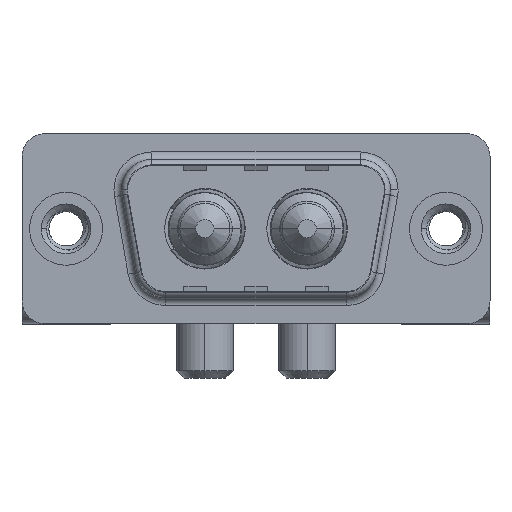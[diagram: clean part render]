
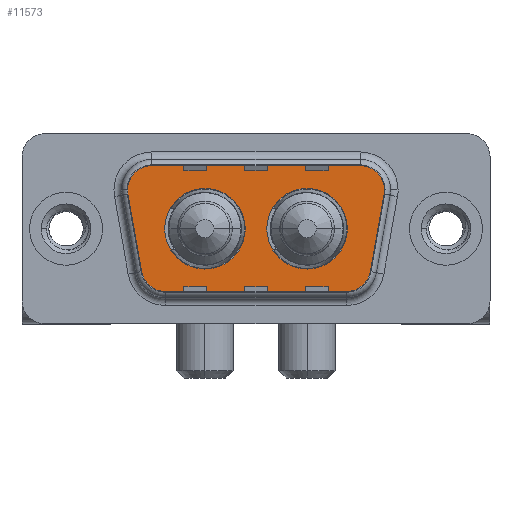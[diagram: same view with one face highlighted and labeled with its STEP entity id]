
A CAD part, top view. The second image highlights one B-rep face of the part: STEP entity #11573.
In plain terms, the highlighted planar face has unit normal (0, 0, 1).
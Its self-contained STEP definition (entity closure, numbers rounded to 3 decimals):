
#195 = EDGE_CURVE ( 'NONE', #11482, #9476, #1524, .T. ) ;
#205 = EDGE_CURVE ( 'NONE', #4298, #3397, #11336, .T. ) ;
#238 = VERTEX_POINT ( 'NONE', #2735 ) ;
#499 = LINE ( 'NONE', #4346, #11280 ) ;
#601 = LINE ( 'NONE', #11205, #11908 ) ;
#615 = LINE ( 'NONE', #6874, #2992 ) ;
#652 = DIRECTION ( 'NONE',  ( 1., 0., 0. ) ) ;
#733 = ORIENTED_EDGE ( 'NONE', *, *, #5882, .T. ) ;
#870 = EDGE_CURVE ( 'NONE', #4586, #8740, #4844, .T. ) ;
#877 = EDGE_LOOP ( 'NONE', ( #5387, #3769 ) ) ;
#968 = EDGE_CURVE ( 'NONE', #10297, #6879, #2413, .T. ) ;
#1195 = ORIENTED_EDGE ( 'NONE', *, *, #8867, .T. ) ;
#1219 = CARTESIAN_POINT ( 'NONE',  ( 5.436, 4.9, 0. ) ) ;
#1524 = LINE ( 'NONE', #3479, #8083 ) ;
#1989 = AXIS2_PLACEMENT_3D ( 'NONE', #2978, #10566, #10689 ) ;
#2013 = CARTESIAN_POINT ( 'NONE',  ( 21.534, 2.553, 0. ) ) ;
#2073 = DIRECTION ( 'NONE',  ( 0., 0., 1. ) ) ;
#2329 = ORIENTED_EDGE ( 'NONE', *, *, #8254, .T. ) ;
#2391 = DIRECTION ( 'NONE',  ( 1., 0., 0. ) ) ;
#2413 = CIRCLE ( 'NONE', #5630, 2.65 ) ;
#2735 = CARTESIAN_POINT ( 'NONE',  ( 6.459, -4.9, 0. ) ) ;
#2789 = ORIENTED_EDGE ( 'NONE', *, *, #870, .F. ) ;
#2978 = CARTESIAN_POINT ( 'NONE',  ( 18.541, -2.9, 0. ) ) ;
#2992 = VECTOR ( 'NONE', #12122, 1000. ) ;
#3397 = VERTEX_POINT ( 'NONE', #11050 ) ;
#3421 = DIRECTION ( 'NONE',  ( 0., 0., 1. ) ) ;
#3461 = DIRECTION ( 'NONE',  ( 0., 0., 1. ) ) ;
#3479 = CARTESIAN_POINT ( 'NONE',  ( 3.466, 2.553, 0. ) ) ;
#3490 = DIRECTION ( 'NONE',  ( 0., 0., 1. ) ) ;
#3769 = ORIENTED_EDGE ( 'NONE', *, *, #9426, .F. ) ;
#3795 = DIRECTION ( 'NONE',  ( 0., 0., 1. ) ) ;
#3797 = FACE_BOUND ( 'NONE', #877, .T. ) ;
#4147 = ORIENTED_EDGE ( 'NONE', *, *, #10955, .F. ) ;
#4204 = AXIS2_PLACEMENT_3D ( 'NONE', #7824, #3795, #8663 ) ;
#4298 = VERTEX_POINT ( 'NONE', #9055 ) ;
#4299 = DIRECTION ( 'NONE',  ( 0., 0., 1. ) ) ;
#4334 = DIRECTION ( 'NONE',  ( 0., 0., 1. ) ) ;
#4346 = CARTESIAN_POINT ( 'NONE',  ( 6.459, -4.9, 0. ) ) ;
#4482 = VERTEX_POINT ( 'NONE', #1219 ) ;
#4558 = CIRCLE ( 'NONE', #5354, 2. ) ;
#4586 = VERTEX_POINT ( 'NONE', #6692 ) ;
#4697 = EDGE_LOOP ( 'NONE', ( #11509, #2329, #8106, #5432, #11906, #733, #9157, #1195, #8414 ) ) ;
#4844 = CIRCLE ( 'NONE', #5446, 2.65 ) ;
#4885 = EDGE_CURVE ( 'NONE', #8788, #11298, #4558, .T. ) ;
#5141 = EDGE_LOOP ( 'NONE', ( #4147, #2789 ) ) ;
#5296 = VERTEX_POINT ( 'NONE', #2013 ) ;
#5308 = DIRECTION ( 'NONE',  ( -1., 0., 0. ) ) ;
#5354 = AXIS2_PLACEMENT_3D ( 'NONE', #10743, #8828, #7877 ) ;
#5387 = ORIENTED_EDGE ( 'NONE', *, *, #968, .F. ) ;
#5432 = ORIENTED_EDGE ( 'NONE', *, *, #4885, .T. ) ;
#5446 = AXIS2_PLACEMENT_3D ( 'NONE', #10741, #2073, #8822 ) ;
#5630 = AXIS2_PLACEMENT_3D ( 'NONE', #7172, #4334, #2391 ) ;
#5875 = CARTESIAN_POINT ( 'NONE',  ( 4.489, -3.247, 0. ) ) ;
#5882 = EDGE_CURVE ( 'NONE', #4482, #11482, #8799, .T. ) ;
#5913 = CARTESIAN_POINT ( 'NONE',  ( 18.51, 0., 0. ) ) ;
#6006 = DIRECTION ( 'NONE',  ( 0., 0., 1. ) ) ;
#6659 = DIRECTION ( 'NONE',  ( -1., 0., 0. ) ) ;
#6692 = CARTESIAN_POINT ( 'NONE',  ( 6.49, 0., 0. ) ) ;
#6874 = CARTESIAN_POINT ( 'NONE',  ( 21.534, 2.553, 0. ) ) ;
#6879 = VERTEX_POINT ( 'NONE', #7616 ) ;
#7172 = CARTESIAN_POINT ( 'NONE',  ( 15.86, 0., 0. ) ) ;
#7276 = CARTESIAN_POINT ( 'NONE',  ( 5.436, 2.9, 0. ) ) ;
#7465 = CARTESIAN_POINT ( 'NONE',  ( 18.541, -2.9, 0. ) ) ;
#7616 = CARTESIAN_POINT ( 'NONE',  ( 13.21, 0., 0. ) ) ;
#7716 = EDGE_CURVE ( 'NONE', #5296, #8788, #10614, .T. ) ;
#7824 = CARTESIAN_POINT ( 'NONE',  ( 15.86, 0., 0. ) ) ;
#7877 = DIRECTION ( 'NONE',  ( -1., 0., 0. ) ) ;
#8015 = CIRCLE ( 'NONE', #8643, 2. ) ;
#8022 = CARTESIAN_POINT ( 'NONE',  ( 19.564, 2.9, 0. ) ) ;
#8083 = VECTOR ( 'NONE', #11137, 1000. ) ;
#8106 = ORIENTED_EDGE ( 'NONE', *, *, #7716, .T. ) ;
#8191 = DIRECTION ( 'NONE',  ( -1., 0., 0. ) ) ;
#8254 = EDGE_CURVE ( 'NONE', #3397, #5296, #615, .T. ) ;
#8260 = CARTESIAN_POINT ( 'NONE',  ( 6.459, -2.9, 0. ) ) ;
#8414 = ORIENTED_EDGE ( 'NONE', *, *, #11818, .T. ) ;
#8422 = DIRECTION ( 'NONE',  ( 1., 0., 0. ) ) ;
#8507 = AXIS2_PLACEMENT_3D ( 'NONE', #7465, #3421, #652 ) ;
#8643 = AXIS2_PLACEMENT_3D ( 'NONE', #8260, #3461, #8191 ) ;
#8663 = DIRECTION ( 'NONE',  ( 1., 0., 0. ) ) ;
#8722 = CARTESIAN_POINT ( 'NONE',  ( 3.466, 2.553, 0. ) ) ;
#8740 = VERTEX_POINT ( 'NONE', #8833 ) ;
#8788 = VERTEX_POINT ( 'NONE', #11756 ) ;
#8799 = CIRCLE ( 'NONE', #10434, 2. ) ;
#8822 = DIRECTION ( 'NONE',  ( 1., 0., 0. ) ) ;
#8828 = DIRECTION ( 'NONE',  ( 0., 0., 1. ) ) ;
#8833 = CARTESIAN_POINT ( 'NONE',  ( 11.79, 0., 0. ) ) ;
#8849 = DIRECTION ( 'NONE',  ( 1., 0., 0. ) ) ;
#8867 = EDGE_CURVE ( 'NONE', #9476, #238, #8015, .T. ) ;
#9055 = CARTESIAN_POINT ( 'NONE',  ( 18.541, -4.9, 0. ) ) ;
#9157 = ORIENTED_EDGE ( 'NONE', *, *, #195, .T. ) ;
#9426 = EDGE_CURVE ( 'NONE', #6879, #10297, #10870, .T. ) ;
#9476 = VERTEX_POINT ( 'NONE', #5875 ) ;
#9653 = CIRCLE ( 'NONE', #11258, 2.65 ) ;
#9687 = FACE_BOUND ( 'NONE', #5141, .T. ) ;
#9794 = PLANE ( 'NONE',  #1989 ) ;
#10172 = DIRECTION ( 'NONE',  ( 1., 0., 0. ) ) ;
#10297 = VERTEX_POINT ( 'NONE', #5913 ) ;
#10434 = AXIS2_PLACEMENT_3D ( 'NONE', #7276, #3490, #8422 ) ;
#10566 = DIRECTION ( 'NONE',  ( 0., 0., 1. ) ) ;
#10614 = CIRCLE ( 'NONE', #12072, 2. ) ;
#10689 = DIRECTION ( 'NONE',  ( 1., 0., 0. ) ) ;
#10741 = CARTESIAN_POINT ( 'NONE',  ( 9.14, 0., 0. ) ) ;
#10743 = CARTESIAN_POINT ( 'NONE',  ( 19.564, 2.9, 0. ) ) ;
#10870 = CIRCLE ( 'NONE', #4204, 2.65 ) ;
#10955 = EDGE_CURVE ( 'NONE', #8740, #4586, #9653, .T. ) ;
#11050 = CARTESIAN_POINT ( 'NONE',  ( 20.511, -3.247, 0. ) ) ;
#11137 = DIRECTION ( 'NONE',  ( 0.174, -0.985, 0. ) ) ;
#11205 = CARTESIAN_POINT ( 'NONE',  ( 5.436, 4.9, 0. ) ) ;
#11252 = CARTESIAN_POINT ( 'NONE',  ( 19.564, 4.9, 0. ) ) ;
#11258 = AXIS2_PLACEMENT_3D ( 'NONE', #11718, #6006, #8849 ) ;
#11280 = VECTOR ( 'NONE', #10172, 1000. ) ;
#11298 = VERTEX_POINT ( 'NONE', #11252 ) ;
#11336 = CIRCLE ( 'NONE', #8507, 2. ) ;
#11482 = VERTEX_POINT ( 'NONE', #8722 ) ;
#11509 = ORIENTED_EDGE ( 'NONE', *, *, #205, .T. ) ;
#11573 = ADVANCED_FACE ( 'NONE', ( #3797, #9687, #11638 ), #9794, .T. ) ;
#11638 = FACE_OUTER_BOUND ( 'NONE', #4697, .T. ) ;
#11718 = CARTESIAN_POINT ( 'NONE',  ( 9.14, 0., 0. ) ) ;
#11756 = CARTESIAN_POINT ( 'NONE',  ( 21.564, 2.9, 0. ) ) ;
#11818 = EDGE_CURVE ( 'NONE', #238, #4298, #499, .T. ) ;
#11906 = ORIENTED_EDGE ( 'NONE', *, *, #12221, .T. ) ;
#11908 = VECTOR ( 'NONE', #6659, 1000. ) ;
#12072 = AXIS2_PLACEMENT_3D ( 'NONE', #8022, #4299, #5308 ) ;
#12122 = DIRECTION ( 'NONE',  ( 0.174, 0.985, 0. ) ) ;
#12221 = EDGE_CURVE ( 'NONE', #11298, #4482, #601, .T. ) ;
